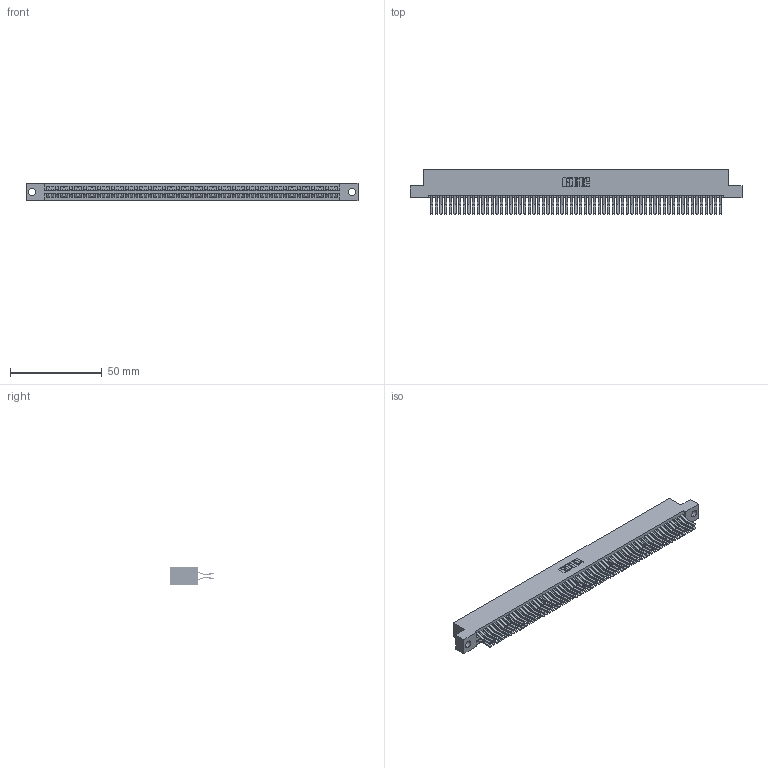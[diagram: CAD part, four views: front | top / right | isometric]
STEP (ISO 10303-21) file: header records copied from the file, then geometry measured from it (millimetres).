
FILE_DESCRIPTION (( 'STEP AP203' ), '1' );
FILE_NAME ('345-126-560-204.STEP', '2021-05-25T19:28:50', ( '' ), ( '' ), 'SwSTEP 2.0', 'SolidWorks 2020', '' );
FILE_SCHEMA (( 'CONFIG_CONTROL_DESIGN' ));
Length unit declared in the file: inch
Products named in the file (3): 345 Part_Flush Mounting Lugs - 0.156 Dia-TI; 345-126-560-204; 345-292-001_560 Tail
Assembly tree (127 placements, depth 2):
  345-126-560-204
    345 Part_Flush Mounting Lugs - 0.156 Dia-TI
    345-292-001_560 Tail  x126
Bounding box: 181.23 x 24.45 x 9.4 mm (x, y, z)
Volume: 18519.6 mm3; surface area: 29757.5 mm2
Topology: 127 solids, 127 shells, 6692 faces, 19907 edges, 13102 vertices
Faces by surface type: plane 4252, cylinder 2440
Entity records: 47111 total; most frequent: CARTESIAN_POINT 7882, ORIENTED_EDGE 7814, DIRECTION 6927, EDGE_CURVE 3907, VECTOR 3519, LINE 3519, VERTEX_POINT 2602, AXIS2_PLACEMENT_3D 1704
